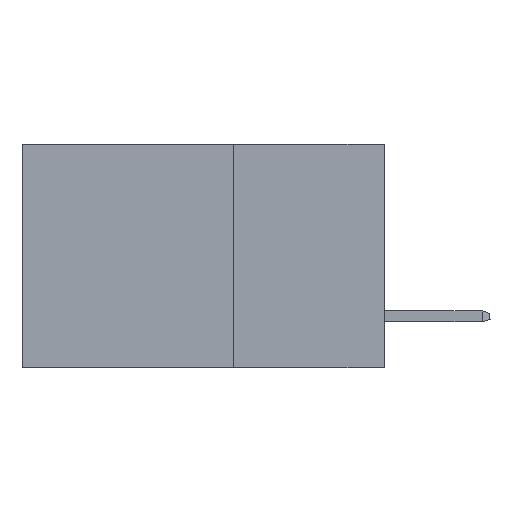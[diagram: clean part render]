
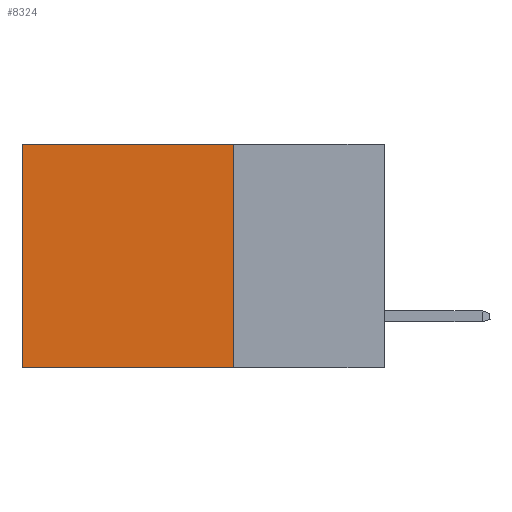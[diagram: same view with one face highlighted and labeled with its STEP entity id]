
A CAD part, left-side view. The second image highlights one B-rep face of the part: STEP entity #8324.
In plain terms, the highlighted planar face has unit normal (-1, 0, 0).
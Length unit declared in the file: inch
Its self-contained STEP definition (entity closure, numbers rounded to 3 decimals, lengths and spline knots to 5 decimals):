
#261 = DIRECTION ( 'NONE',  ( 0., 0., -1. ) ) ;
#1515 = DIRECTION ( 'NONE',  ( 1., 0., 0. ) ) ;
#1573 = LINE ( 'NONE', #7767, #10899 ) ;
#1929 = CARTESIAN_POINT ( 'NONE',  ( 0.298, 0.6, 0. ) ) ;
#2054 = DIRECTION ( 'NONE',  ( 0., 0., -1. ) ) ;
#2316 = CARTESIAN_POINT ( 'NONE',  ( 0.298, 0.25, 0. ) ) ;
#2862 = EDGE_CURVE ( 'NONE', #3807, #6879, #7924, .T. ) ;
#3202 = CARTESIAN_POINT ( 'NONE',  ( 0.298, 0.6, 0. ) ) ;
#3767 = VERTEX_POINT ( 'NONE', #1929 ) ;
#3807 = VERTEX_POINT ( 'NONE', #4853 ) ;
#3872 = EDGE_CURVE ( 'NONE', #3767, #6879, #9825, .T. ) ;
#3904 = ORIENTED_EDGE ( 'NONE', *, *, #3872, .T. ) ;
#4070 = AXIS2_PLACEMENT_3D ( 'NONE', #2316, #1515, #8026 ) ;
#4181 = VECTOR ( 'NONE', #2054, 39.37008 ) ;
#4785 = DIRECTION ( 'NONE',  ( 0., 1., 0. ) ) ;
#4853 = CARTESIAN_POINT ( 'NONE',  ( 0.298, 0.25, -0.37 ) ) ;
#4862 = CARTESIAN_POINT ( 'NONE',  ( 0.298, 0.6, -0.37 ) ) ;
#4941 = ORIENTED_EDGE ( 'NONE', *, *, #8931, .F. ) ;
#5041 = FACE_OUTER_BOUND ( 'NONE', #7764, .T. ) ;
#5215 = DIRECTION ( 'NONE',  ( 0., 1., 0. ) ) ;
#5429 = VECTOR ( 'NONE', #5215, 39.37008 ) ;
#6106 = VERTEX_POINT ( 'NONE', #8952 ) ;
#6137 = ORIENTED_EDGE ( 'NONE', *, *, #6460, .T. ) ;
#6460 = EDGE_CURVE ( 'NONE', #6106, #3767, #1573, .T. ) ;
#6879 = VERTEX_POINT ( 'NONE', #4862 ) ;
#7318 = VECTOR ( 'NONE', #261, 39.37008 ) ;
#7764 = EDGE_LOOP ( 'NONE', ( #3904, #12100, #4941, #6137 ) ) ;
#7767 = CARTESIAN_POINT ( 'NONE',  ( 0.298, 0.25, 0. ) ) ;
#7924 = LINE ( 'NONE', #11830, #5429 ) ;
#8026 = DIRECTION ( 'NONE',  ( 0., 0., -1. ) ) ;
#8324 = ADVANCED_FACE ( 'NONE', ( #5041 ), #9075, .F. ) ;
#8650 = CARTESIAN_POINT ( 'NONE',  ( 0.298, 0.25, 0. ) ) ;
#8931 = EDGE_CURVE ( 'NONE', #6106, #3807, #11565, .T. ) ;
#8952 = CARTESIAN_POINT ( 'NONE',  ( 0.298, 0.25, 0. ) ) ;
#9075 = PLANE ( 'NONE',  #4070 ) ;
#9825 = LINE ( 'NONE', #3202, #7318 ) ;
#10899 = VECTOR ( 'NONE', #4785, 39.37008 ) ;
#11565 = LINE ( 'NONE', #8650, #4181 ) ;
#11830 = CARTESIAN_POINT ( 'NONE',  ( 0.298, 0.25, -0.37 ) ) ;
#12100 = ORIENTED_EDGE ( 'NONE', *, *, #2862, .F. ) ;
